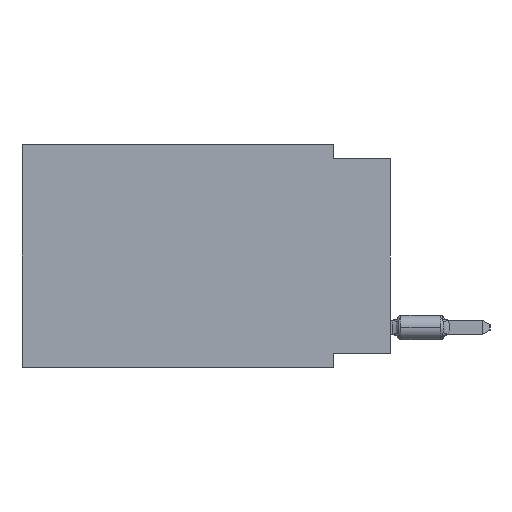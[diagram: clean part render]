
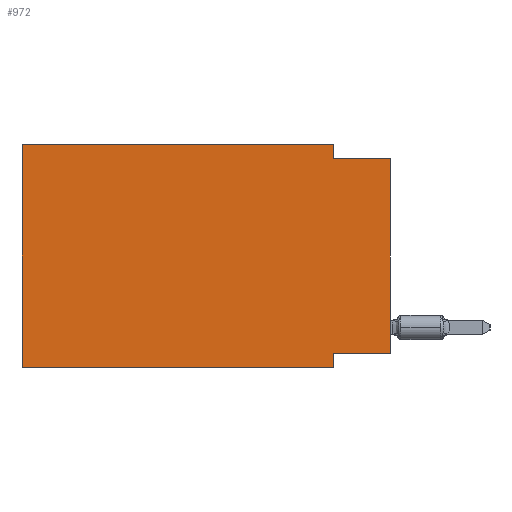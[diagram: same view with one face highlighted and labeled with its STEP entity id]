
A CAD part, left-side view. The second image highlights one B-rep face of the part: STEP entity #972.
In plain terms, the highlighted planar face has unit normal (-1, 0, 0).
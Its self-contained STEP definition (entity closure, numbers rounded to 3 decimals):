
#159 = ORIENTED_EDGE ( 'NONE', *, *, #27327, .F. ) ;
#224 = CARTESIAN_POINT ( 'NONE',  ( 0., 0., -0.635 ) ) ;
#972 = ADVANCED_FACE ( 'NONE', ( #23892 ), #1971, .F. ) ;
#1971 = PLANE ( 'NONE',  #6373 ) ;
#2565 = CARTESIAN_POINT ( 'NONE',  ( 0., 16.383, 0. ) ) ;
#2600 = ORIENTED_EDGE ( 'NONE', *, *, #33231, .F. ) ;
#2729 = EDGE_CURVE ( 'NONE', #37859, #28633, #32920, .T. ) ;
#2766 = ORIENTED_EDGE ( 'NONE', *, *, #25064, .T. ) ;
#3436 = CARTESIAN_POINT ( 'NONE',  ( 0., 2.54, 0. ) ) ;
#3736 = CARTESIAN_POINT ( 'NONE',  ( 0., 2.54, -9.271 ) ) ;
#4106 = VERTEX_POINT ( 'NONE', #33941 ) ;
#5693 = ORIENTED_EDGE ( 'NONE', *, *, #37040, .F. ) ;
#6155 = LINE ( 'NONE', #27309, #35630 ) ;
#6373 = AXIS2_PLACEMENT_3D ( 'NONE', #2565, #20650, #21255 ) ;
#6427 = LINE ( 'NONE', #12133, #24745 ) ;
#6588 = EDGE_CURVE ( 'NONE', #10528, #38178, #6427, .T. ) ;
#7103 = LINE ( 'NONE', #26013, #24303 ) ;
#7794 = ORIENTED_EDGE ( 'NONE', *, *, #2729, .F. ) ;
#9180 = DIRECTION ( 'NONE',  ( 0., 0., -1. ) ) ;
#9364 = LINE ( 'NONE', #24822, #16150 ) ;
#10341 = VECTOR ( 'NONE', #9180, 1000. ) ;
#10528 = VERTEX_POINT ( 'NONE', #3736 ) ;
#10739 = VERTEX_POINT ( 'NONE', #12228 ) ;
#11687 = VECTOR ( 'NONE', #17462, 1000. ) ;
#12034 = LINE ( 'NONE', #33378, #10341 ) ;
#12133 = CARTESIAN_POINT ( 'NONE',  ( 0., 2.54, -9.906 ) ) ;
#12228 = CARTESIAN_POINT ( 'NONE',  ( 0., 0., -9.271 ) ) ;
#13513 = CARTESIAN_POINT ( 'NONE',  ( 0., 16.383, 0. ) ) ;
#14372 = CARTESIAN_POINT ( 'NONE',  ( 0., 16.383, -9.906 ) ) ;
#16150 = VECTOR ( 'NONE', #18715, 1000. ) ;
#16924 = VERTEX_POINT ( 'NONE', #13513 ) ;
#17062 = DIRECTION ( 'NONE',  ( 0., 0., 1. ) ) ;
#17462 = DIRECTION ( 'NONE',  ( 0., -1., 0. ) ) ;
#18144 = ORIENTED_EDGE ( 'NONE', *, *, #33790, .F. ) ;
#18428 = CARTESIAN_POINT ( 'NONE',  ( 0., 2.54, -0.635 ) ) ;
#18715 = DIRECTION ( 'NONE',  ( 0., 0., 1. ) ) ;
#19964 = EDGE_CURVE ( 'NONE', #10739, #28633, #7103, .T. ) ;
#20142 = ORIENTED_EDGE ( 'NONE', *, *, #6588, .F. ) ;
#20650 = DIRECTION ( 'NONE',  ( 1., 0., 0. ) ) ;
#20847 = ORIENTED_EDGE ( 'NONE', *, *, #19964, .T. ) ;
#20868 = LINE ( 'NONE', #14372, #35498 ) ;
#21255 = DIRECTION ( 'NONE',  ( 0., 0., -1. ) ) ;
#22292 = DIRECTION ( 'NONE',  ( 0., 0., -1. ) ) ;
#22548 = LINE ( 'NONE', #34943, #23845 ) ;
#22978 = CARTESIAN_POINT ( 'NONE',  ( 0., 0., -0.635 ) ) ;
#23471 = CARTESIAN_POINT ( 'NONE',  ( 0., 2.54, -9.906 ) ) ;
#23540 = EDGE_LOOP ( 'NONE', ( #20847, #7794, #159, #2600, #5693, #2766, #20142, #18144 ) ) ;
#23845 = VECTOR ( 'NONE', #37389, 1000. ) ;
#23892 = FACE_OUTER_BOUND ( 'NONE', #23540, .T. ) ;
#24303 = VECTOR ( 'NONE', #17062, 1000. ) ;
#24745 = VECTOR ( 'NONE', #22292, 1000. ) ;
#24822 = CARTESIAN_POINT ( 'NONE',  ( 0., 16.383, 0. ) ) ;
#25064 = EDGE_CURVE ( 'NONE', #4106, #38178, #20868, .T. ) ;
#26013 = CARTESIAN_POINT ( 'NONE',  ( 0., 0., 0. ) ) ;
#26063 = VERTEX_POINT ( 'NONE', #3436 ) ;
#26774 = DIRECTION ( 'NONE',  ( 0., -1., 0. ) ) ;
#27309 = CARTESIAN_POINT ( 'NONE',  ( 0., 16.383, 0. ) ) ;
#27327 = EDGE_CURVE ( 'NONE', #26063, #37859, #12034, .T. ) ;
#28633 = VERTEX_POINT ( 'NONE', #224 ) ;
#32920 = LINE ( 'NONE', #22978, #11687 ) ;
#33231 = EDGE_CURVE ( 'NONE', #16924, #26063, #6155, .T. ) ;
#33378 = CARTESIAN_POINT ( 'NONE',  ( 0., 2.54, 0. ) ) ;
#33790 = EDGE_CURVE ( 'NONE', #10739, #10528, #22548, .T. ) ;
#33941 = CARTESIAN_POINT ( 'NONE',  ( 0., 16.383, -9.906 ) ) ;
#34943 = CARTESIAN_POINT ( 'NONE',  ( 0., 0., -9.271 ) ) ;
#35498 = VECTOR ( 'NONE', #26774, 1000. ) ;
#35630 = VECTOR ( 'NONE', #39704, 1000. ) ;
#37040 = EDGE_CURVE ( 'NONE', #4106, #16924, #9364, .T. ) ;
#37389 = DIRECTION ( 'NONE',  ( 0., 1., 0. ) ) ;
#37859 = VERTEX_POINT ( 'NONE', #18428 ) ;
#38178 = VERTEX_POINT ( 'NONE', #23471 ) ;
#39704 = DIRECTION ( 'NONE',  ( 0., -1., 0. ) ) ;
